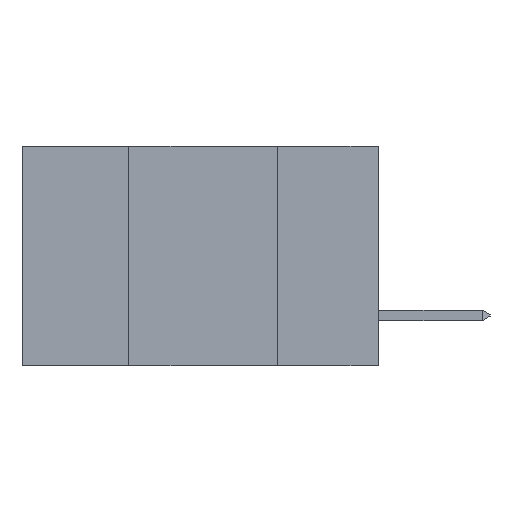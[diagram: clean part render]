
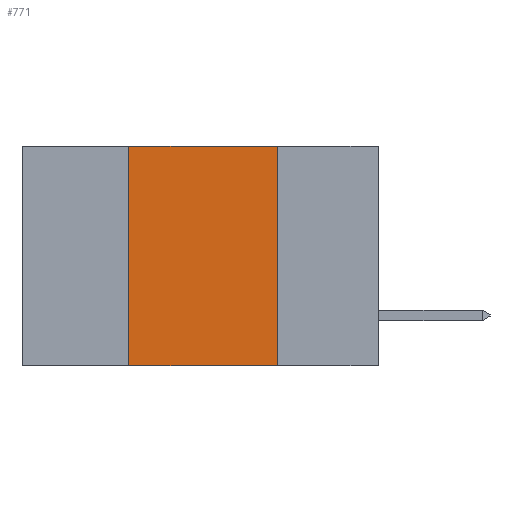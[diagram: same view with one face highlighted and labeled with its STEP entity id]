
A CAD part, left-side view. The second image highlights one B-rep face of the part: STEP entity #771.
In plain terms, the highlighted planar face has unit normal (-1, 0, 0).
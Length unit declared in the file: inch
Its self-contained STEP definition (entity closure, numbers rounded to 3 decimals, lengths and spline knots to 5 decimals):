
#349 = ORIENTED_EDGE ( 'NONE', *, *, #5899, .F. ) ;
#771 = ADVANCED_FACE ( 'NONE', ( #6209 ), #2283, .F. ) ;
#1211 = CARTESIAN_POINT ( 'NONE',  ( 0., 0.17, -0.37 ) ) ;
#1661 = CARTESIAN_POINT ( 'NONE',  ( 0., 0.6, 0. ) ) ;
#1760 = VERTEX_POINT ( 'NONE', #7521 ) ;
#1830 = DIRECTION ( 'NONE',  ( 0., 0., -1. ) ) ;
#2283 = PLANE ( 'NONE',  #11894 ) ;
#2411 = DIRECTION ( 'NONE',  ( 0., -1., 0. ) ) ;
#2821 = VERTEX_POINT ( 'NONE', #8688 ) ;
#3842 = EDGE_CURVE ( 'NONE', #4282, #2821, #11331, .T. ) ;
#4282 = VERTEX_POINT ( 'NONE', #7982 ) ;
#4324 = EDGE_LOOP ( 'NONE', ( #4796, #6109, #349, #4884 ) ) ;
#4796 = ORIENTED_EDGE ( 'NONE', *, *, #9019, .F. ) ;
#4884 = ORIENTED_EDGE ( 'NONE', *, *, #3842, .T. ) ;
#4917 = LINE ( 'NONE', #11887, #11921 ) ;
#5081 = LINE ( 'NONE', #10840, #12073 ) ;
#5232 = EDGE_CURVE ( 'NONE', #1760, #10682, #5081, .T. ) ;
#5899 = EDGE_CURVE ( 'NONE', #4282, #1760, #4917, .T. ) ;
#5955 = DIRECTION ( 'NONE',  ( 1., 0., 0. ) ) ;
#6109 = ORIENTED_EDGE ( 'NONE', *, *, #5232, .F. ) ;
#6209 = FACE_OUTER_BOUND ( 'NONE', #4324, .T. ) ;
#7254 = DIRECTION ( 'NONE',  ( 0., 0., -1. ) ) ;
#7521 = CARTESIAN_POINT ( 'NONE',  ( 0., 0.42, 0. ) ) ;
#7982 = CARTESIAN_POINT ( 'NONE',  ( 0., 0.42, -0.37 ) ) ;
#8277 = CARTESIAN_POINT ( 'NONE',  ( 0., 0.17, 0. ) ) ;
#8688 = CARTESIAN_POINT ( 'NONE',  ( 0., 0.17, -0.37 ) ) ;
#9019 = EDGE_CURVE ( 'NONE', #10682, #2821, #12244, .T. ) ;
#9120 = VECTOR ( 'NONE', #2411, 39.37008 ) ;
#9430 = CARTESIAN_POINT ( 'NONE',  ( 0., 0.6, -0.37 ) ) ;
#9796 = VECTOR ( 'NONE', #7254, 39.37008 ) ;
#9964 = DIRECTION ( 'NONE',  ( 0., -1., 0. ) ) ;
#10682 = VERTEX_POINT ( 'NONE', #8277 ) ;
#10840 = CARTESIAN_POINT ( 'NONE',  ( 0., 0.6, 0. ) ) ;
#11331 = LINE ( 'NONE', #9430, #9120 ) ;
#11841 = DIRECTION ( 'NONE',  ( 0., 0., 1. ) ) ;
#11887 = CARTESIAN_POINT ( 'NONE',  ( 0., 0.42, -0.37 ) ) ;
#11894 = AXIS2_PLACEMENT_3D ( 'NONE', #1661, #5955, #1830 ) ;
#11921 = VECTOR ( 'NONE', #11841, 39.37008 ) ;
#12073 = VECTOR ( 'NONE', #9964, 39.37008 ) ;
#12244 = LINE ( 'NONE', #1211, #9796 ) ;
